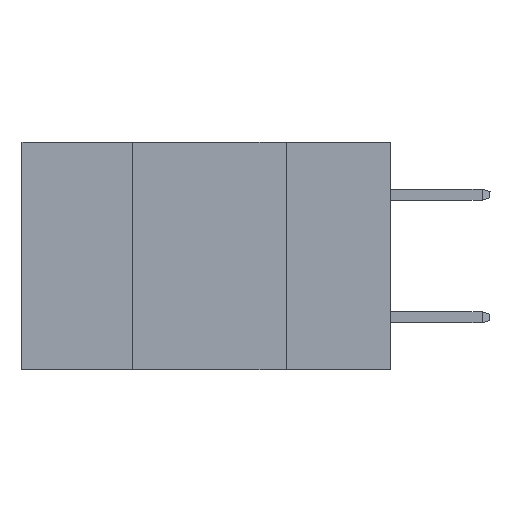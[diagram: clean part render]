
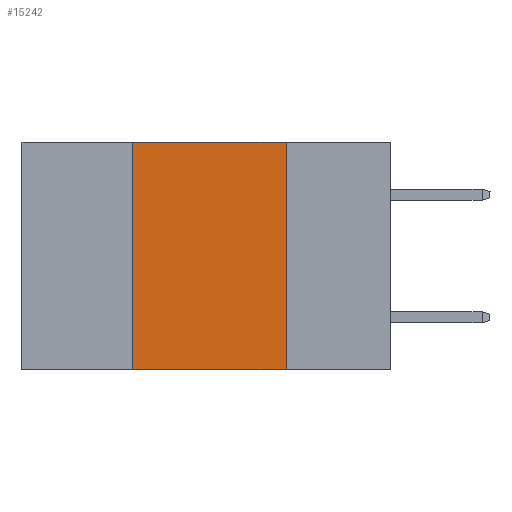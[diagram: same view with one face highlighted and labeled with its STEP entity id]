
A CAD part, left-side view. The second image highlights one B-rep face of the part: STEP entity #15242.
In plain terms, the highlighted planar face has unit normal (-1, 0, 0).
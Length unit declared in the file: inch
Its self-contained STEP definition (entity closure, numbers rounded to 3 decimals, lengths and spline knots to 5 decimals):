
#209 = CARTESIAN_POINT ( 'NONE',  ( 0., 0.17, 0. ) ) ;
#362 = ORIENTED_EDGE ( 'NONE', *, *, #18626, .T. ) ;
#537 = CARTESIAN_POINT ( 'NONE',  ( 0., 0.6, 0. ) ) ;
#610 = EDGE_LOOP ( 'NONE', ( #12572, #10499, #8713, #362 ) ) ;
#1843 = CARTESIAN_POINT ( 'NONE',  ( 0., 0.42, 0. ) ) ;
#2563 = DIRECTION ( 'NONE',  ( 0., 0., -1. ) ) ;
#3374 = DIRECTION ( 'NONE',  ( 0., 0., -1. ) ) ;
#3626 = VECTOR ( 'NONE', #12901, 39.37008 ) ;
#4033 = AXIS2_PLACEMENT_3D ( 'NONE', #537, #14178, #2563 ) ;
#4828 = VERTEX_POINT ( 'NONE', #209 ) ;
#5316 = VERTEX_POINT ( 'NONE', #24662 ) ;
#5506 = VERTEX_POINT ( 'NONE', #7953 ) ;
#5896 = DIRECTION ( 'NONE',  ( 0., 0., 1. ) ) ;
#6031 = LINE ( 'NONE', #14981, #16204 ) ;
#6568 = VERTEX_POINT ( 'NONE', #1843 ) ;
#7237 = VECTOR ( 'NONE', #5896, 39.37008 ) ;
#7953 = CARTESIAN_POINT ( 'NONE',  ( 0., 0.17, -0.37 ) ) ;
#8713 = ORIENTED_EDGE ( 'NONE', *, *, #21963, .F. ) ;
#10333 = PLANE ( 'NONE',  #4033 ) ;
#10499 = ORIENTED_EDGE ( 'NONE', *, *, #17437, .F. ) ;
#12129 = LINE ( 'NONE', #12370, #22087 ) ;
#12370 = CARTESIAN_POINT ( 'NONE',  ( 0., 0.6, -0.37 ) ) ;
#12572 = ORIENTED_EDGE ( 'NONE', *, *, #20167, .F. ) ;
#12901 = DIRECTION ( 'NONE',  ( 0., -1., 0. ) ) ;
#14178 = DIRECTION ( 'NONE',  ( 1., 0., 0. ) ) ;
#14981 = CARTESIAN_POINT ( 'NONE',  ( 0., 0.17, 0. ) ) ;
#15242 = ADVANCED_FACE ( 'NONE', ( #18472 ), #10333, .F. ) ;
#16204 = VECTOR ( 'NONE', #3374, 39.37008 ) ;
#17358 = LINE ( 'NONE', #19210, #7237 ) ;
#17437 = EDGE_CURVE ( 'NONE', #6568, #4828, #18931, .T. ) ;
#18472 = FACE_OUTER_BOUND ( 'NONE', #610, .T. ) ;
#18626 = EDGE_CURVE ( 'NONE', #5316, #5506, #12129, .T. ) ;
#18931 = LINE ( 'NONE', #20381, #3626 ) ;
#19210 = CARTESIAN_POINT ( 'NONE',  ( 0., 0.42, 0. ) ) ;
#19936 = DIRECTION ( 'NONE',  ( 0., -1., 0. ) ) ;
#20167 = EDGE_CURVE ( 'NONE', #4828, #5506, #6031, .T. ) ;
#20381 = CARTESIAN_POINT ( 'NONE',  ( 0., 0.6, 0. ) ) ;
#21963 = EDGE_CURVE ( 'NONE', #5316, #6568, #17358, .T. ) ;
#22087 = VECTOR ( 'NONE', #19936, 39.37008 ) ;
#24662 = CARTESIAN_POINT ( 'NONE',  ( 0., 0.42, -0.37 ) ) ;
